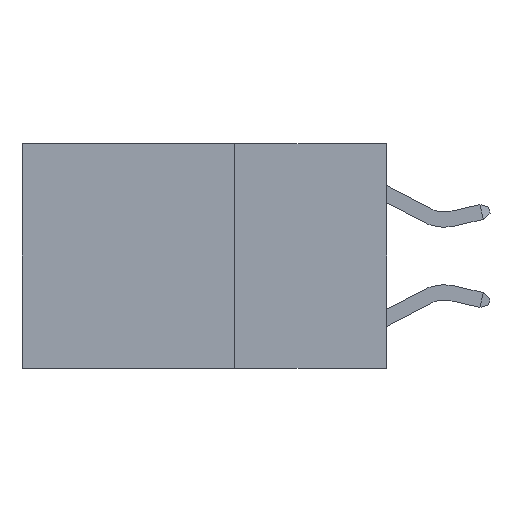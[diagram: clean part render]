
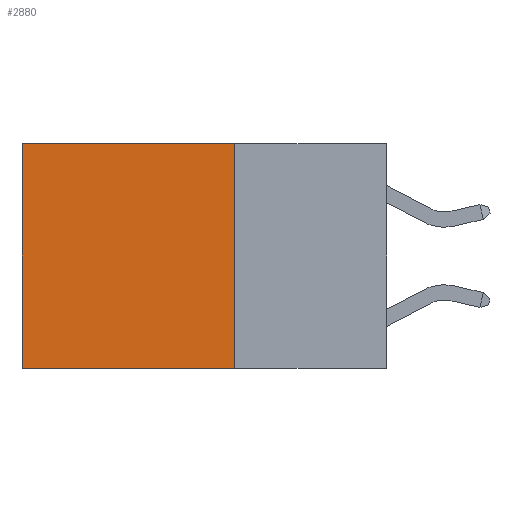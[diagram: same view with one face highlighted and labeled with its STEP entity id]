
A CAD part, left-side view. The second image highlights one B-rep face of the part: STEP entity #2880.
In plain terms, the highlighted planar face has unit normal (-1, 0, 0).
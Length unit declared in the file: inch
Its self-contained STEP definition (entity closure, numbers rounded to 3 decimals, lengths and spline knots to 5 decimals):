
#605 = VECTOR ( 'NONE', #4046, 39.37008 ) ;
#943 = LINE ( 'NONE', #7399, #4963 ) ;
#1698 = FACE_OUTER_BOUND ( 'NONE', #3748, .T. ) ;
#1760 = VECTOR ( 'NONE', #3731, 39.37008 ) ;
#2353 = ORIENTED_EDGE ( 'NONE', *, *, #7138, .T. ) ;
#2389 = ORIENTED_EDGE ( 'NONE', *, *, #2939, .F. ) ;
#2502 = ORIENTED_EDGE ( 'NONE', *, *, #9158, .F. ) ;
#2523 = ORIENTED_EDGE ( 'NONE', *, *, #6804, .T. ) ;
#2590 = VERTEX_POINT ( 'NONE', #5395 ) ;
#2880 = ADVANCED_FACE ( 'NONE', ( #1698 ), #4644, .F. ) ;
#2939 = EDGE_CURVE ( 'NONE', #4231, #2590, #943, .T. ) ;
#3288 = DIRECTION ( 'NONE',  ( 0., 0., -1. ) ) ;
#3731 = DIRECTION ( 'NONE',  ( 0., 1., 0. ) ) ;
#3748 = EDGE_LOOP ( 'NONE', ( #2353, #2389, #2502, #2523 ) ) ;
#3782 = CARTESIAN_POINT ( 'NONE',  ( 0.2625, 0.25, 0. ) ) ;
#3873 = LINE ( 'NONE', #8305, #1760 ) ;
#3924 = CARTESIAN_POINT ( 'NONE',  ( 0.2625, 0.6, 0. ) ) ;
#3975 = CARTESIAN_POINT ( 'NONE',  ( 0.2625, 0.25, 0. ) ) ;
#4046 = DIRECTION ( 'NONE',  ( 0., 0., -1. ) ) ;
#4231 = VERTEX_POINT ( 'NONE', #6020 ) ;
#4644 = PLANE ( 'NONE',  #7766 ) ;
#4744 = DIRECTION ( 'NONE',  ( 0., 0., -1. ) ) ;
#4963 = VECTOR ( 'NONE', #7363, 39.37008 ) ;
#4993 = DIRECTION ( 'NONE',  ( 1., 0., 0. ) ) ;
#5123 = LINE ( 'NONE', #6369, #605 ) ;
#5395 = CARTESIAN_POINT ( 'NONE',  ( 0.2625, 0.6, -0.37 ) ) ;
#6020 = CARTESIAN_POINT ( 'NONE',  ( 0.2625, 0.25, -0.37 ) ) ;
#6369 = CARTESIAN_POINT ( 'NONE',  ( 0.2625, 0.25, 0. ) ) ;
#6688 = LINE ( 'NONE', #7241, #8676 ) ;
#6804 = EDGE_CURVE ( 'NONE', #7054, #7573, #3873, .T. ) ;
#7054 = VERTEX_POINT ( 'NONE', #3975 ) ;
#7138 = EDGE_CURVE ( 'NONE', #7573, #2590, #6688, .T. ) ;
#7241 = CARTESIAN_POINT ( 'NONE',  ( 0.2625, 0.6, 0. ) ) ;
#7363 = DIRECTION ( 'NONE',  ( 0., 1., 0. ) ) ;
#7399 = CARTESIAN_POINT ( 'NONE',  ( 0.2625, 0.25, -0.37 ) ) ;
#7573 = VERTEX_POINT ( 'NONE', #3924 ) ;
#7766 = AXIS2_PLACEMENT_3D ( 'NONE', #3782, #4993, #4744 ) ;
#8305 = CARTESIAN_POINT ( 'NONE',  ( 0.2625, 0.25, 0. ) ) ;
#8676 = VECTOR ( 'NONE', #3288, 39.37008 ) ;
#9158 = EDGE_CURVE ( 'NONE', #7054, #4231, #5123, .T. ) ;
